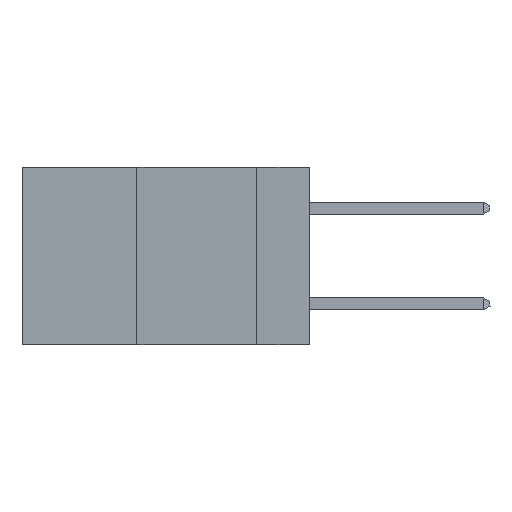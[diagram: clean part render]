
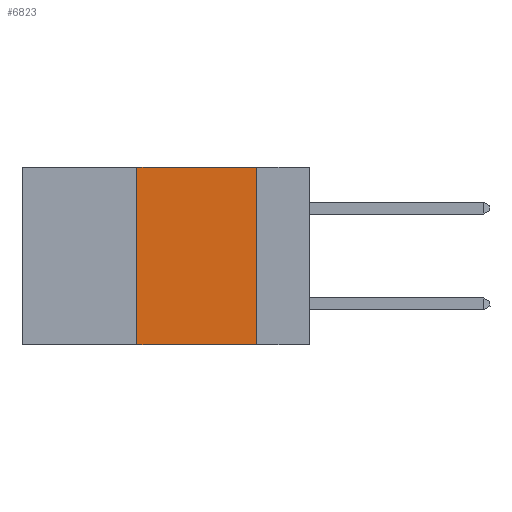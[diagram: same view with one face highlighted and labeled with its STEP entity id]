
A CAD part, left-side view. The second image highlights one B-rep face of the part: STEP entity #6823.
In plain terms, the highlighted planar face has unit normal (-1, 0, 0).
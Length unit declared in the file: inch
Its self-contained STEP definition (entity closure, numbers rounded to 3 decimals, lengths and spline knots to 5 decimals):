
#270 = CARTESIAN_POINT ( 'NONE',  ( 0., 0.6, 0. ) ) ;
#640 = VERTEX_POINT ( 'NONE', #2267 ) ;
#807 = EDGE_CURVE ( 'NONE', #11102, #640, #12611, .T. ) ;
#1151 = CARTESIAN_POINT ( 'NONE',  ( 0., 0.11, 0. ) ) ;
#1192 = LINE ( 'NONE', #11181, #9511 ) ;
#1553 = ORIENTED_EDGE ( 'NONE', *, *, #807, .T. ) ;
#2086 = EDGE_CURVE ( 'NONE', #9115, #2899, #2459, .T. ) ;
#2110 = CARTESIAN_POINT ( 'NONE',  ( 0., 0.6, 0. ) ) ;
#2267 = CARTESIAN_POINT ( 'NONE',  ( 0., 0.11, -0.37 ) ) ;
#2459 = LINE ( 'NONE', #2110, #11129 ) ;
#2484 = CARTESIAN_POINT ( 'NONE',  ( 0., 0.11, 0. ) ) ;
#2899 = VERTEX_POINT ( 'NONE', #1151 ) ;
#3504 = PLANE ( 'NONE',  #7006 ) ;
#3979 = ORIENTED_EDGE ( 'NONE', *, *, #9726, .F. ) ;
#4255 = VECTOR ( 'NONE', #7517, 39.37008 ) ;
#4623 = DIRECTION ( 'NONE',  ( 0., 0., -1. ) ) ;
#5054 = DIRECTION ( 'NONE',  ( 0., -1., 0. ) ) ;
#5147 = EDGE_CURVE ( 'NONE', #11102, #9115, #1192, .T. ) ;
#5351 = CARTESIAN_POINT ( 'NONE',  ( 0., 0.6, -0.37 ) ) ;
#5685 = DIRECTION ( 'NONE',  ( 0., 0., -1. ) ) ;
#6512 = CARTESIAN_POINT ( 'NONE',  ( 0., 0.36, 0. ) ) ;
#6766 = ORIENTED_EDGE ( 'NONE', *, *, #5147, .F. ) ;
#6823 = ADVANCED_FACE ( 'NONE', ( #12585 ), #3504, .F. ) ;
#7006 = AXIS2_PLACEMENT_3D ( 'NONE', #270, #7297, #4623 ) ;
#7297 = DIRECTION ( 'NONE',  ( 1., 0., 0. ) ) ;
#7517 = DIRECTION ( 'NONE',  ( 0., -1., 0. ) ) ;
#7915 = DIRECTION ( 'NONE',  ( 0., 0., 1. ) ) ;
#9115 = VERTEX_POINT ( 'NONE', #6512 ) ;
#9511 = VECTOR ( 'NONE', #7915, 39.37008 ) ;
#9546 = CARTESIAN_POINT ( 'NONE',  ( 0., 0.36, -0.37 ) ) ;
#9547 = ORIENTED_EDGE ( 'NONE', *, *, #2086, .F. ) ;
#9726 = EDGE_CURVE ( 'NONE', #2899, #640, #9895, .T. ) ;
#9895 = LINE ( 'NONE', #2484, #11706 ) ;
#10398 = EDGE_LOOP ( 'NONE', ( #3979, #9547, #6766, #1553 ) ) ;
#11102 = VERTEX_POINT ( 'NONE', #9546 ) ;
#11129 = VECTOR ( 'NONE', #5054, 39.37008 ) ;
#11181 = CARTESIAN_POINT ( 'NONE',  ( 0., 0.36, 0. ) ) ;
#11706 = VECTOR ( 'NONE', #5685, 39.37008 ) ;
#12585 = FACE_OUTER_BOUND ( 'NONE', #10398, .T. ) ;
#12611 = LINE ( 'NONE', #5351, #4255 ) ;
